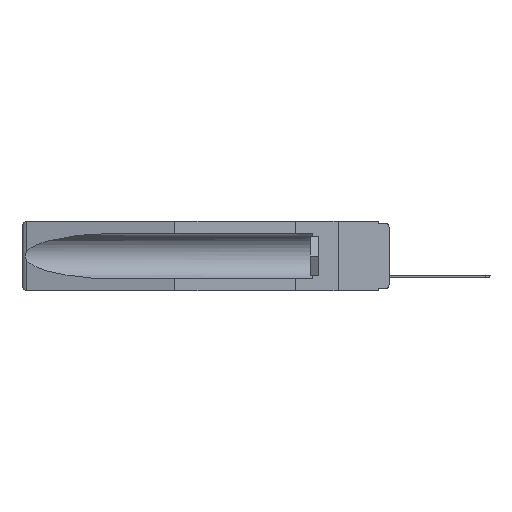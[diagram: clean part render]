
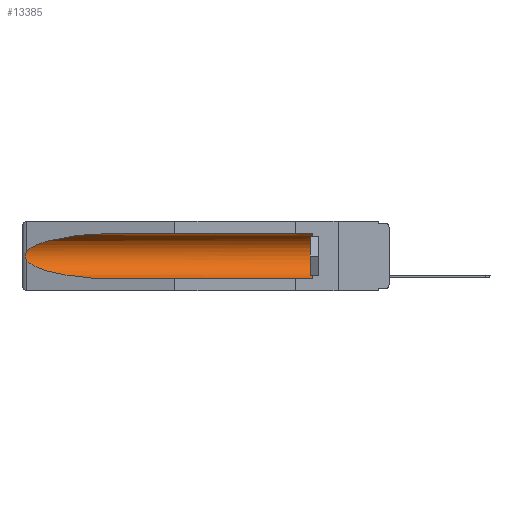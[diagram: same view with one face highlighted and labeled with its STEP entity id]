
A CAD part, left-side view. The second image highlights one B-rep face of the part: STEP entity #13385.
In plain terms, the highlighted cylindrical face has radius 2.857 mm (diameter 5.715 mm), a partial arc.
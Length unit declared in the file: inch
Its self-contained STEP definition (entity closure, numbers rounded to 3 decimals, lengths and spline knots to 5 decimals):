
#180 = VERTEX_POINT ( 'NONE', #4383 ) ;
#868 = FACE_OUTER_BOUND ( 'NONE', #1456, .T. ) ;
#1456 = EDGE_LOOP ( 'NONE', ( #8812, #8648, #25507, #11914, #22459, #5758 ) ) ;
#1821 = VERTEX_POINT ( 'NONE', #17457 ) ;
#3579 = CARTESIAN_POINT ( 'NONE',  ( 0.2673, 1.5327, -0.16383 ) ) ;
#4383 = CARTESIAN_POINT ( 'NONE',  ( 0.155, 1.07973, -0.059 ) ) ;
#5308 = CARTESIAN_POINT ( 'NONE',  ( 0.155, 1.07973, -0.284 ) ) ;
#5758 = ORIENTED_EDGE ( 'NONE', *, *, #12512, .T. ) ;
#7298 = VERTEX_POINT ( 'NONE', #21842 ) ;
#7707 = EDGE_CURVE ( 'NONE', #180, #1821, #21417, .T. ) ;
#8648 = ORIENTED_EDGE ( 'NONE', *, *, #21525, .T. ) ;
#8694 = CARTESIAN_POINT ( 'NONE',  ( 0.155, 0.126, -0.1715 ) ) ;
#8812 = ORIENTED_EDGE ( 'NONE', *, *, #7707, .T. ) ;
#9387 = CARTESIAN_POINT ( 'NONE',  ( 0.26537, 1.52718, -0.19328 ) ) ;
#9738 = VERTEX_POINT ( 'NONE', #17166 ) ;
#9835 = CARTESIAN_POINT ( 'NONE',  ( 0.2675, 1.53308, -0.16763 ) ) ;
#9923 = CARTESIAN_POINT ( 'NONE',  ( 0.155, 1.07973, -0.059 ) ) ;
#10193 = CARTESIAN_POINT ( 'NONE',  ( 0.155, -0.30754, -0.284 ) ) ;
#10953 = DIRECTION ( 'NONE',  ( 0., 0., 1. ) ) ;
#11836 = DIRECTION ( 'NONE',  ( 0., 0., 1. ) ) ;
#11872 = CARTESIAN_POINT ( 'NONE',  ( 0.21114, 1.30732, -0.284 ) ) ;
#11914 = ORIENTED_EDGE ( 'NONE', *, *, #17823, .F. ) ;
#12071 = CARTESIAN_POINT ( 'NONE',  ( 0.21114, 1.30732, -0.059 ) ) ;
#12115 = CARTESIAN_POINT ( 'NONE',  ( 0.26537, 1.52718, -0.14972 ) ) ;
#12251 = CARTESIAN_POINT ( 'NONE',  ( 0.2673, 1.53269, -0.17917 ) ) ;
#12512 = EDGE_CURVE ( 'NONE', #9738, #180, #18329, .T. ) ;
#13385 = ADVANCED_FACE ( 'NONE', ( #868 ), #18263, .F. ) ;
#14117 = DIRECTION ( 'NONE',  ( 0., 1., 0. ) ) ;
#14252 = CARTESIAN_POINT ( 'NONE',  ( 0.26655, 1.53094, -0.18657 ) ) ;
#14348 = VECTOR ( 'NONE', #16752, 39.37008 ) ;
#14468 = LINE ( 'NONE', #10193, #14348 ) ;
#14818 =( BOUNDED_CURVE ( )  B_SPLINE_CURVE ( 3, ( #26329, #20299, #11872, #27270 ),
 .UNSPECIFIED., .F., .F. ) 
 B_SPLINE_CURVE_WITH_KNOTS ( ( 4, 4 ),
 ( 0.1948, 1.5708 ),
 .UNSPECIFIED. ) 
 CURVE ( )  GEOMETRIC_REPRESENTATION_ITEM ( )  RATIONAL_B_SPLINE_CURVE ( ( 1., 0.848, 0.848, 1. ) ) 
 REPRESENTATION_ITEM ( '' )  );
#16110 = CARTESIAN_POINT ( 'NONE',  ( 0.155, -0.30754, -0.1715 ) ) ;
#16752 = DIRECTION ( 'NONE',  ( 0., 1., 0. ) ) ;
#16807 = CARTESIAN_POINT ( 'NONE',  ( 0.26597, 1.5296, -0.19026 ) ) ;
#17166 = CARTESIAN_POINT ( 'NONE',  ( 0.155, 0.126, -0.059 ) ) ;
#17241 = DIRECTION ( 'NONE',  ( 0., -1., 0. ) ) ;
#17457 = CARTESIAN_POINT ( 'NONE',  ( 0.26537, 1.52718, -0.14972 ) ) ;
#17823 = EDGE_CURVE ( 'NONE', #7298, #18517, #14468, .T. ) ;
#18263 = CYLINDRICAL_SURFACE ( 'NONE', #26518, 0.1125 ) ;
#18329 = LINE ( 'NONE', #27300, #23306 ) ;
#18517 = VERTEX_POINT ( 'NONE', #5308 ) ;
#18625 = CARTESIAN_POINT ( 'NONE',  ( 0.26537, 1.52718, -0.14972 ) ) ;
#19619 = CIRCLE ( 'NONE', #23716, 0.1125 ) ;
#20299 = CARTESIAN_POINT ( 'NONE',  ( 0.25451, 1.48313, -0.24835 ) ) ;
#20740 = B_SPLINE_CURVE_WITH_KNOTS ( 'NONE', 3,
 ( #12115, #20813, #25377, #3579, #9835, #25100, #12251, #14252, #16807, #21242 ),
 .UNSPECIFIED., .F., .F.,
 ( 4, 2, 2, 2, 4 ),
 ( 0., 0.00029, 0.00058, 0.00087, 0.00117 ),
 .UNSPECIFIED. ) ;
#20813 = CARTESIAN_POINT ( 'NONE',  ( 0.26597, 1.52961, -0.15275 ) ) ;
#21242 = CARTESIAN_POINT ( 'NONE',  ( 0.26537, 1.52718, -0.19328 ) ) ;
#21417 =( BOUNDED_CURVE ( )  B_SPLINE_CURVE ( 3, ( #9923, #12071, #27049, #18625 ),
 .UNSPECIFIED., .F., .T. ) 
 B_SPLINE_CURVE_WITH_KNOTS ( ( 4, 4 ),
 ( 4.71239, 6.08839 ),
 .UNSPECIFIED. ) 
 CURVE ( )  GEOMETRIC_REPRESENTATION_ITEM ( )  RATIONAL_B_SPLINE_CURVE ( ( 1., 0.848, 0.848, 1. ) ) 
 REPRESENTATION_ITEM ( '' )  );
#21525 = EDGE_CURVE ( 'NONE', #1821, #26610, #20740, .T. ) ;
#21842 = CARTESIAN_POINT ( 'NONE',  ( 0.155, 0.126, -0.284 ) ) ;
#22228 = EDGE_CURVE ( 'NONE', #26610, #18517, #14818, .T. ) ;
#22459 = ORIENTED_EDGE ( 'NONE', *, *, #27786, .T. ) ;
#23306 = VECTOR ( 'NONE', #27026, 39.37008 ) ;
#23716 = AXIS2_PLACEMENT_3D ( 'NONE', #8694, #17241, #10953 ) ;
#25100 = CARTESIAN_POINT ( 'NONE',  ( 0.2675, 1.53308, -0.17534 ) ) ;
#25377 = CARTESIAN_POINT ( 'NONE',  ( 0.26654, 1.53092, -0.15636 ) ) ;
#25507 = ORIENTED_EDGE ( 'NONE', *, *, #22228, .T. ) ;
#26329 = CARTESIAN_POINT ( 'NONE',  ( 0.26537, 1.52718, -0.19328 ) ) ;
#26518 = AXIS2_PLACEMENT_3D ( 'NONE', #16110, #14117, #11836 ) ;
#26610 = VERTEX_POINT ( 'NONE', #9387 ) ;
#27026 = DIRECTION ( 'NONE',  ( 0., 1., 0. ) ) ;
#27049 = CARTESIAN_POINT ( 'NONE',  ( 0.25451, 1.48313, -0.09465 ) ) ;
#27270 = CARTESIAN_POINT ( 'NONE',  ( 0.155, 1.07973, -0.284 ) ) ;
#27300 = CARTESIAN_POINT ( 'NONE',  ( 0.155, -0.30754, -0.059 ) ) ;
#27786 = EDGE_CURVE ( 'NONE', #7298, #9738, #19619, .T. ) ;
